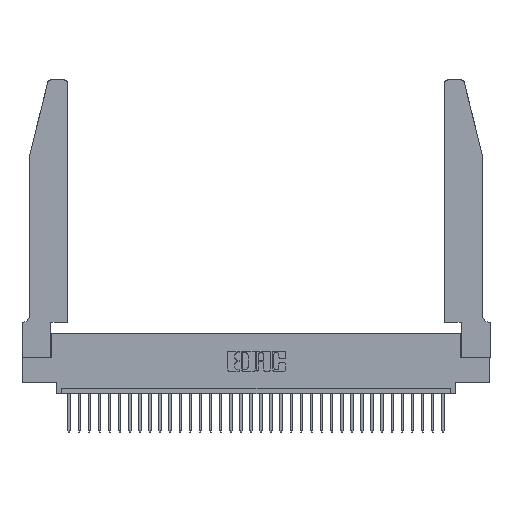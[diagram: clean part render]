
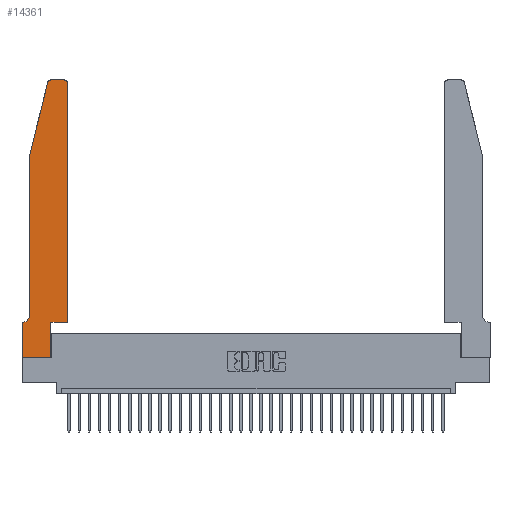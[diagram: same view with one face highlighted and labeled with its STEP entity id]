
A CAD part, top view. The second image highlights one B-rep face of the part: STEP entity #14361.
In plain terms, the highlighted planar face has unit normal (0, 0, 1).
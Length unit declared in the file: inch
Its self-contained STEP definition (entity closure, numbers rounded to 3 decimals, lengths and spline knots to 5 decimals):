
#442 = CARTESIAN_POINT ( 'NONE',  ( 0.0055, 0.42, 0.37 ) ) ;
#472 = VERTEX_POINT ( 'NONE', #9714 ) ;
#1463 = CIRCLE ( 'NONE', #5237, 0.07 ) ;
#1743 = ORIENTED_EDGE ( 'NONE', *, *, #8508, .T. ) ;
#2061 = EDGE_CURVE ( 'NONE', #21790, #21734, #18495, .T. ) ;
#2073 = CARTESIAN_POINT ( 'NONE',  ( 0.4205, 2.72, 0.37 ) ) ;
#2429 = ORIENTED_EDGE ( 'NONE', *, *, #27007, .T. ) ;
#2434 = VECTOR ( 'NONE', #4586, 39.37008 ) ;
#2653 = AXIS2_PLACEMENT_3D ( 'NONE', #33871, #33534, #31352 ) ;
#2657 = ORIENTED_EDGE ( 'NONE', *, *, #3887, .T. ) ;
#2884 = LINE ( 'NONE', #11119, #10285 ) ;
#2917 = CIRCLE ( 'NONE', #2653, 0.03 ) ;
#3314 = EDGE_CURVE ( 'NONE', #31072, #14604, #2917, .T. ) ;
#3423 = ORIENTED_EDGE ( 'NONE', *, *, #3314, .T. ) ;
#3887 = EDGE_CURVE ( 'NONE', #472, #31072, #2884, .T. ) ;
#4423 = EDGE_LOOP ( 'NONE', ( #2657, #3423, #30913, #2429, #28437, #21869, #29863, #28217, #21171, #7636, #18319, #1743 ) ) ;
#4457 = CARTESIAN_POINT ( 'NONE',  ( 0.4505, 0.35, 0.37 ) ) ;
#4586 = DIRECTION ( 'NONE',  ( 0., -1., 0. ) ) ;
#4872 = EDGE_CURVE ( 'NONE', #15996, #26947, #12264, .T. ) ;
#4950 = FACE_OUTER_BOUND ( 'NONE', #4423, .T. ) ;
#5156 = CARTESIAN_POINT ( 'NONE',  ( 0.2865, 0.35, 0.37 ) ) ;
#5184 = AXIS2_PLACEMENT_3D ( 'NONE', #2073, #20110, #17596 ) ;
#5237 = AXIS2_PLACEMENT_3D ( 'NONE', #442, #29182, #31854 ) ;
#5957 = CARTESIAN_POINT ( 'NONE',  ( 0., 0.35, 0.37 ) ) ;
#6005 = VERTEX_POINT ( 'NONE', #14712 ) ;
#7609 = LINE ( 'NONE', #27181, #11693 ) ;
#7636 = ORIENTED_EDGE ( 'NONE', *, *, #31542, .T. ) ;
#8167 = DIRECTION ( 'NONE',  ( 1., 0., 0. ) ) ;
#8177 = CARTESIAN_POINT ( 'NONE',  ( 0., 0.35, 0.37 ) ) ;
#8273 = VECTOR ( 'NONE', #13810, 39.37008 ) ;
#8508 = EDGE_CURVE ( 'NONE', #16345, #472, #27728, .T. ) ;
#8627 = EDGE_CURVE ( 'NONE', #14604, #26058, #7609, .T. ) ;
#9714 = CARTESIAN_POINT ( 'NONE',  ( 0.4205, 2.75, 0.37 ) ) ;
#10285 = VECTOR ( 'NONE', #31590, 39.37008 ) ;
#10309 = CARTESIAN_POINT ( 'NONE',  ( 0., 0., 0.37 ) ) ;
#11119 = CARTESIAN_POINT ( 'NONE',  ( 0.2605, 2.75, 0.37 ) ) ;
#11693 = VECTOR ( 'NONE', #24392, 39.37008 ) ;
#12264 = LINE ( 'NONE', #28360, #2434 ) ;
#13443 = DIRECTION ( 'NONE',  ( 1., 0., 0. ) ) ;
#13810 = DIRECTION ( 'NONE',  ( 0., 1., 0. ) ) ;
#14303 = DIRECTION ( 'NONE',  ( -1., 0., 0. ) ) ;
#14361 = ADVANCED_FACE ( 'NONE', ( #4950 ), #18673, .T. ) ;
#14604 = VERTEX_POINT ( 'NONE', #17489 ) ;
#14712 = CARTESIAN_POINT ( 'NONE',  ( 0.0755, 0.42, 0.37 ) ) ;
#14884 = VECTOR ( 'NONE', #32513, 39.37008 ) ;
#15827 = CARTESIAN_POINT ( 'NONE',  ( 0.4505, 0.35, 0.37 ) ) ;
#15996 = VERTEX_POINT ( 'NONE', #5957 ) ;
#16128 = CARTESIAN_POINT ( 'NONE',  ( 0., 0., 0.37 ) ) ;
#16205 = VECTOR ( 'NONE', #31367, 39.37008 ) ;
#16345 = VERTEX_POINT ( 'NONE', #21584 ) ;
#16373 = VERTEX_POINT ( 'NONE', #19168 ) ;
#17489 = CARTESIAN_POINT ( 'NONE',  ( 0.25487, 2.72718, 0.37 ) ) ;
#17596 = DIRECTION ( 'NONE',  ( 1., 0., 0. ) ) ;
#18263 = VERTEX_POINT ( 'NONE', #18750 ) ;
#18319 = ORIENTED_EDGE ( 'NONE', *, *, #23329, .T. ) ;
#18495 = LINE ( 'NONE', #33982, #8273 ) ;
#18673 = PLANE ( 'NONE',  #31501 ) ;
#18750 = CARTESIAN_POINT ( 'NONE',  ( 0.4505, 0.35, 0.37 ) ) ;
#19168 = CARTESIAN_POINT ( 'NONE',  ( 0.0055, 0.35, 0.37 ) ) ;
#19182 = CARTESIAN_POINT ( 'NONE',  ( 0.0755, 0.35, 0.37 ) ) ;
#20110 = DIRECTION ( 'NONE',  ( 0., 0., 1. ) ) ;
#21171 = ORIENTED_EDGE ( 'NONE', *, *, #2061, .T. ) ;
#21223 = CARTESIAN_POINT ( 'NONE',  ( 0.2865, 0., 0.37 ) ) ;
#21316 = DIRECTION ( 'NONE',  ( 0., 0., 1. ) ) ;
#21465 = VECTOR ( 'NONE', #14303, 39.37008 ) ;
#21584 = CARTESIAN_POINT ( 'NONE',  ( 0.4505, 2.72, 0.37 ) ) ;
#21734 = VERTEX_POINT ( 'NONE', #5156 ) ;
#21790 = VERTEX_POINT ( 'NONE', #21223 ) ;
#21869 = ORIENTED_EDGE ( 'NONE', *, *, #23209, .T. ) ;
#22368 = EDGE_CURVE ( 'NONE', #6005, #16373, #1463, .T. ) ;
#22759 = LINE ( 'NONE', #19182, #21465 ) ;
#22998 = DIRECTION ( 'NONE',  ( 0., 1., 0. ) ) ;
#23209 = EDGE_CURVE ( 'NONE', #16373, #15996, #22759, .T. ) ;
#23329 = EDGE_CURVE ( 'NONE', #18263, #16345, #24821, .T. ) ;
#23586 = VECTOR ( 'NONE', #22998, 39.37008 ) ;
#23991 = LINE ( 'NONE', #15827, #31077 ) ;
#24392 = DIRECTION ( 'NONE',  ( -0.239, -0.971, 0. ) ) ;
#24821 = LINE ( 'NONE', #4457, #23586 ) ;
#24946 = CARTESIAN_POINT ( 'NONE',  ( 0.0755, 2., 0.37 ) ) ;
#26058 = VERTEX_POINT ( 'NONE', #24946 ) ;
#26947 = VERTEX_POINT ( 'NONE', #16128 ) ;
#27007 = EDGE_CURVE ( 'NONE', #26058, #6005, #31759, .T. ) ;
#27181 = CARTESIAN_POINT ( 'NONE',  ( 0.0755, 2., 0.37 ) ) ;
#27728 = CIRCLE ( 'NONE', #5184, 0.03 ) ;
#27802 = LINE ( 'NONE', #10309, #16205 ) ;
#28217 = ORIENTED_EDGE ( 'NONE', *, *, #30877, .T. ) ;
#28360 = CARTESIAN_POINT ( 'NONE',  ( 0., 0., 0.37 ) ) ;
#28437 = ORIENTED_EDGE ( 'NONE', *, *, #22368, .T. ) ;
#29182 = DIRECTION ( 'NONE',  ( 0., 0., -1. ) ) ;
#29863 = ORIENTED_EDGE ( 'NONE', *, *, #4872, .T. ) ;
#30877 = EDGE_CURVE ( 'NONE', #26947, #21790, #27802, .T. ) ;
#30913 = ORIENTED_EDGE ( 'NONE', *, *, #8627, .T. ) ;
#31072 = VERTEX_POINT ( 'NONE', #32342 ) ;
#31077 = VECTOR ( 'NONE', #8167, 39.37008 ) ;
#31352 = DIRECTION ( 'NONE',  ( 1., 0., 0. ) ) ;
#31367 = DIRECTION ( 'NONE',  ( 1., 0., 0. ) ) ;
#31501 = AXIS2_PLACEMENT_3D ( 'NONE', #8177, #21316, #13443 ) ;
#31542 = EDGE_CURVE ( 'NONE', #21734, #18263, #23991, .T. ) ;
#31590 = DIRECTION ( 'NONE',  ( -1., 0., 0. ) ) ;
#31759 = LINE ( 'NONE', #32189, #14884 ) ;
#31854 = DIRECTION ( 'NONE',  ( -1., 0., 0. ) ) ;
#32189 = CARTESIAN_POINT ( 'NONE',  ( 0.0755, 2., 0.37 ) ) ;
#32342 = CARTESIAN_POINT ( 'NONE',  ( 0.284, 2.75, 0.37 ) ) ;
#32513 = DIRECTION ( 'NONE',  ( 0., -1., 0. ) ) ;
#33534 = DIRECTION ( 'NONE',  ( 0., 0., 1. ) ) ;
#33871 = CARTESIAN_POINT ( 'NONE',  ( 0.284, 2.72, 0.37 ) ) ;
#33982 = CARTESIAN_POINT ( 'NONE',  ( 0.2865, 0.35, 0.37 ) ) ;
